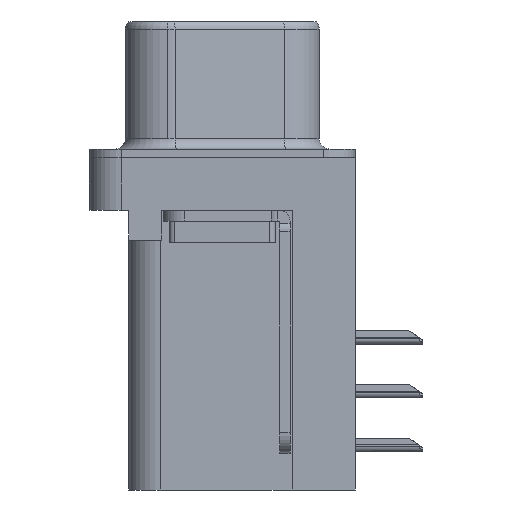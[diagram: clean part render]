
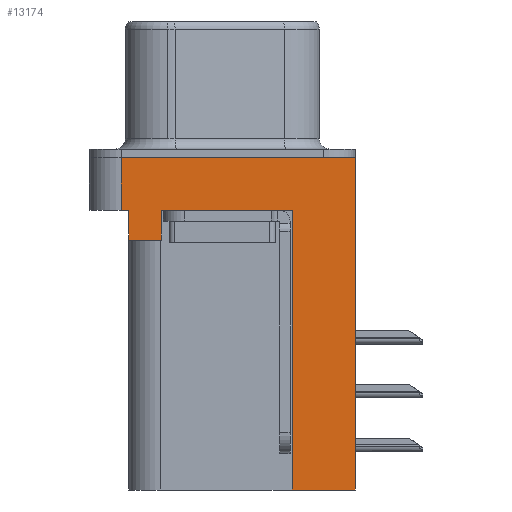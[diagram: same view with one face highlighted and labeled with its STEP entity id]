
A CAD part, left-side view. The second image highlights one B-rep face of the part: STEP entity #13174.
In plain terms, the highlighted planar face has unit normal (-1, 0, 0).
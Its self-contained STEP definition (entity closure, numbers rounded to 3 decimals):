
#141 = LINE ( 'NONE', #18044, #866 ) ;
#288 = FACE_OUTER_BOUND ( 'NONE', #2452, .T. ) ;
#308 = DIRECTION ( 'NONE',  ( 0., -1., 0. ) ) ;
#653 = EDGE_CURVE ( 'NONE', #18830, #28056, #13018, .T. ) ;
#789 = ORIENTED_EDGE ( 'NONE', *, *, #9347, .T. ) ;
#793 = VECTOR ( 'NONE', #23997, 1000. ) ;
#862 = CARTESIAN_POINT ( 'NONE',  ( -3., 4.425, -3.9 ) ) ;
#866 = VECTOR ( 'NONE', #27175, 1000. ) ;
#1046 = ORIENTED_EDGE ( 'NONE', *, *, #9228, .F. ) ;
#1668 = VECTOR ( 'NONE', #27633, 1000. ) ;
#2364 = CARTESIAN_POINT ( 'NONE',  ( -3., -6.275, -2.5 ) ) ;
#2452 = EDGE_LOOP ( 'NONE', ( #2679, #25759, #26855, #1046, #8078, #9329, #789, #17494, #15189, #23907 ) ) ;
#2559 = VERTEX_POINT ( 'NONE', #19897 ) ;
#2679 = ORIENTED_EDGE ( 'NONE', *, *, #19118, .F. ) ;
#3636 = VECTOR ( 'NONE', #16185, 1000. ) ;
#3688 = LINE ( 'NONE', #26876, #20407 ) ;
#3697 = CARTESIAN_POINT ( 'NONE',  ( -3., 4.775, 0. ) ) ;
#3930 = DIRECTION ( 'NONE',  ( 0., 1., 0. ) ) ;
#3981 = CARTESIAN_POINT ( 'NONE',  ( -3., 4.425, -3.9 ) ) ;
#4680 = DIRECTION ( 'NONE',  ( -1., 0., 0. ) ) ;
#5671 = LINE ( 'NONE', #15532, #29232 ) ;
#6836 = LINE ( 'NONE', #8040, #793 ) ;
#7401 = VERTEX_POINT ( 'NONE', #9536 ) ;
#8040 = CARTESIAN_POINT ( 'NONE',  ( -3., 2.895, -3.9 ) ) ;
#8078 = ORIENTED_EDGE ( 'NONE', *, *, #11217, .F. ) ;
#8185 = CARTESIAN_POINT ( 'NONE',  ( -3., 4.775, -2.5 ) ) ;
#9228 = EDGE_CURVE ( 'NONE', #15962, #24205, #3688, .T. ) ;
#9329 = ORIENTED_EDGE ( 'NONE', *, *, #22640, .T. ) ;
#9347 = EDGE_CURVE ( 'NONE', #13447, #28056, #141, .T. ) ;
#9536 = CARTESIAN_POINT ( 'NONE',  ( -3., -6.275, -15.7 ) ) ;
#10570 = EDGE_CURVE ( 'NONE', #23438, #12382, #17104, .T. ) ;
#11090 = VECTOR ( 'NONE', #17289, 1000. ) ;
#11217 = EDGE_CURVE ( 'NONE', #2559, #15962, #15673, .T. ) ;
#12057 = VECTOR ( 'NONE', #3930, 1000. ) ;
#12382 = VERTEX_POINT ( 'NONE', #3697 ) ;
#12502 = EDGE_CURVE ( 'NONE', #23438, #24205, #5671, .T. ) ;
#13018 = LINE ( 'NONE', #20040, #1668 ) ;
#13105 = DIRECTION ( 'NONE',  ( 0., 1., 0. ) ) ;
#13174 = ADVANCED_FACE ( 'NONE', ( #288 ), #18237, .T. ) ;
#13192 = DIRECTION ( 'NONE',  ( 0., 0., 1. ) ) ;
#13447 = VERTEX_POINT ( 'NONE', #14491 ) ;
#13910 = CARTESIAN_POINT ( 'NONE',  ( -3., -6.275, 0. ) ) ;
#14491 = CARTESIAN_POINT ( 'NONE',  ( -3., 2.895, -2.5 ) ) ;
#14960 = VECTOR ( 'NONE', #13105, 1000. ) ;
#15022 = LINE ( 'NONE', #16082, #3636 ) ;
#15189 = ORIENTED_EDGE ( 'NONE', *, *, #20045, .F. ) ;
#15224 = CARTESIAN_POINT ( 'NONE',  ( -3., -3.295, -15.7 ) ) ;
#15249 = CARTESIAN_POINT ( 'NONE',  ( -3., -3.295, -15.7 ) ) ;
#15532 = CARTESIAN_POINT ( 'NONE',  ( -3., -6.275, -2.5 ) ) ;
#15673 = LINE ( 'NONE', #3981, #14960 ) ;
#15962 = VERTEX_POINT ( 'NONE', #862 ) ;
#16082 = CARTESIAN_POINT ( 'NONE',  ( -3., -6.275, -2.5 ) ) ;
#16185 = DIRECTION ( 'NONE',  ( 0., 0., 1. ) ) ;
#16591 = EDGE_CURVE ( 'NONE', #7401, #24818, #15022, .T. ) ;
#17104 = LINE ( 'NONE', #8185, #11090 ) ;
#17289 = DIRECTION ( 'NONE',  ( 0., 0., 1. ) ) ;
#17494 = ORIENTED_EDGE ( 'NONE', *, *, #653, .F. ) ;
#18044 = CARTESIAN_POINT ( 'NONE',  ( -3., -6.275, -2.5 ) ) ;
#18237 = PLANE ( 'NONE',  #23102 ) ;
#18830 = VERTEX_POINT ( 'NONE', #15224 ) ;
#19118 = EDGE_CURVE ( 'NONE', #12382, #24818, #27449, .T. ) ;
#19897 = CARTESIAN_POINT ( 'NONE',  ( -3., 2.895, -3.9 ) ) ;
#20040 = CARTESIAN_POINT ( 'NONE',  ( -3., -3.295, -15.7 ) ) ;
#20045 = EDGE_CURVE ( 'NONE', #7401, #18830, #24113, .T. ) ;
#20407 = VECTOR ( 'NONE', #13192, 1000. ) ;
#20555 = DIRECTION ( 'NONE',  ( 0., 0., 1. ) ) ;
#21334 = VECTOR ( 'NONE', #308, 1000. ) ;
#22463 = CARTESIAN_POINT ( 'NONE',  ( -3., 4.775, -2.5 ) ) ;
#22640 = EDGE_CURVE ( 'NONE', #2559, #13447, #6836, .T. ) ;
#23102 = AXIS2_PLACEMENT_3D ( 'NONE', #2364, #4680, #20555 ) ;
#23438 = VERTEX_POINT ( 'NONE', #22463 ) ;
#23824 = CARTESIAN_POINT ( 'NONE',  ( -3., -3.295, -2.5 ) ) ;
#23907 = ORIENTED_EDGE ( 'NONE', *, *, #16591, .T. ) ;
#23997 = DIRECTION ( 'NONE',  ( 0., 0., 1. ) ) ;
#24113 = LINE ( 'NONE', #15249, #12057 ) ;
#24205 = VERTEX_POINT ( 'NONE', #28700 ) ;
#24684 = DIRECTION ( 'NONE',  ( 0., -1., 0. ) ) ;
#24818 = VERTEX_POINT ( 'NONE', #28257 ) ;
#25759 = ORIENTED_EDGE ( 'NONE', *, *, #10570, .F. ) ;
#26855 = ORIENTED_EDGE ( 'NONE', *, *, #12502, .T. ) ;
#26876 = CARTESIAN_POINT ( 'NONE',  ( -3., 4.425, -3.9 ) ) ;
#27175 = DIRECTION ( 'NONE',  ( 0., -1., 0. ) ) ;
#27449 = LINE ( 'NONE', #13910, #21334 ) ;
#27633 = DIRECTION ( 'NONE',  ( 0., 0., 1. ) ) ;
#28056 = VERTEX_POINT ( 'NONE', #23824 ) ;
#28257 = CARTESIAN_POINT ( 'NONE',  ( -3., -6.275, 0. ) ) ;
#28700 = CARTESIAN_POINT ( 'NONE',  ( -3., 4.425, -2.5 ) ) ;
#29232 = VECTOR ( 'NONE', #24684, 1000. ) ;
